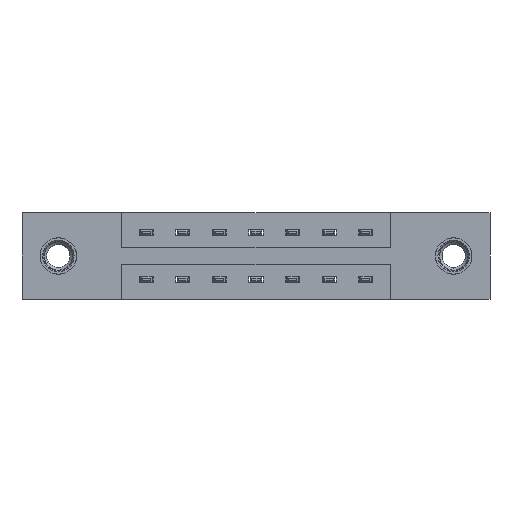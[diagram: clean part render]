
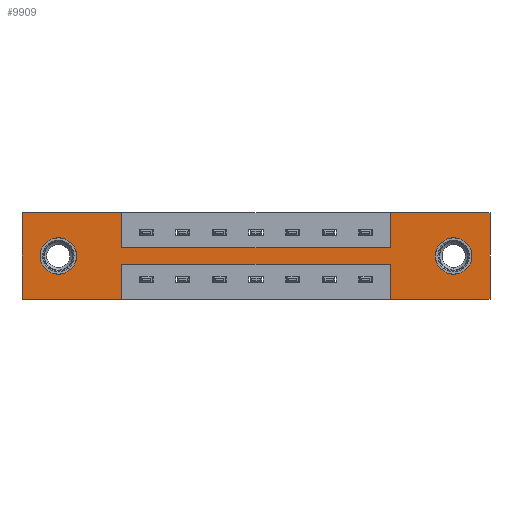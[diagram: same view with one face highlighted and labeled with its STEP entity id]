
A CAD part, front view. The second image highlights one B-rep face of the part: STEP entity #9909.
In plain terms, the highlighted planar face has unit normal (0, -1, 0).
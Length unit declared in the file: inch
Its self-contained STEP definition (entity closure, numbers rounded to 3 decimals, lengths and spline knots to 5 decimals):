
#42 = CARTESIAN_POINT ( 'NONE',  ( 0.425, 0., 0. ) ) ;
#105 = CARTESIAN_POINT ( 'NONE',  ( 1.843, 0., -0.263 ) ) ;
#265 = DIRECTION ( 'NONE',  ( 0., 0., 1. ) ) ;
#335 = DIRECTION ( 'NONE',  ( 0., 0., -1. ) ) ;
#348 = CARTESIAN_POINT ( 'NONE',  ( 0., 0., 0. ) ) ;
#365 = FACE_BOUND ( 'NONE', #8200, .T. ) ;
#426 = LINE ( 'NONE', #6497, #5454 ) ;
#581 = DIRECTION ( 'NONE',  ( 0., 0., 1. ) ) ;
#606 = EDGE_CURVE ( 'NONE', #2423, #4986, #8933, .T. ) ;
#896 = FACE_BOUND ( 'NONE', #5640, .T. ) ;
#1083 = VECTOR ( 'NONE', #9210, 39.37008 ) ;
#1389 = EDGE_CURVE ( 'NONE', #10096, #5776, #8411, .T. ) ;
#1401 = VERTEX_POINT ( 'NONE', #105 ) ;
#1419 = DIRECTION ( 'NONE',  ( 0., 0., -1. ) ) ;
#1502 = VECTOR ( 'NONE', #4473, 39.37008 ) ;
#1526 = CARTESIAN_POINT ( 'NONE',  ( 1.573, 0., -0.37 ) ) ;
#1586 = DIRECTION ( 'NONE',  ( 0., 1., 0. ) ) ;
#1689 = DIRECTION ( 'NONE',  ( 0., 0., -1. ) ) ;
#1734 = DIRECTION ( 'NONE',  ( 0., -1., 0. ) ) ;
#1774 = VERTEX_POINT ( 'NONE', #4088 ) ;
#1817 = PLANE ( 'NONE',  #8766 ) ;
#2056 = DIRECTION ( 'NONE',  ( -1., 0., 0. ) ) ;
#2137 = LINE ( 'NONE', #7655, #5462 ) ;
#2291 = EDGE_CURVE ( 'NONE', #4266, #7596, #2137, .T. ) ;
#2322 = CIRCLE ( 'NONE', #10658, 0.078 ) ;
#2397 = CARTESIAN_POINT ( 'NONE',  ( 0., 0., -0.37 ) ) ;
#2423 = VERTEX_POINT ( 'NONE', #4426 ) ;
#2525 = DIRECTION ( 'NONE',  ( 1., 0., 0. ) ) ;
#2531 = ORIENTED_EDGE ( 'NONE', *, *, #10396, .T. ) ;
#2560 = CARTESIAN_POINT ( 'NONE',  ( 0., 0., -0.37 ) ) ;
#2608 = EDGE_CURVE ( 'NONE', #10381, #10036, #426, .T. ) ;
#2638 = CARTESIAN_POINT ( 'NONE',  ( 1.843, 0., -0.185 ) ) ;
#2710 = ORIENTED_EDGE ( 'NONE', *, *, #8866, .T. ) ;
#2764 = CARTESIAN_POINT ( 'NONE',  ( 0., 0., -0.37 ) ) ;
#2765 = EDGE_CURVE ( 'NONE', #7596, #10561, #3045, .T. ) ;
#2774 = LINE ( 'NONE', #3293, #1083 ) ;
#2861 = FACE_OUTER_BOUND ( 'NONE', #7091, .T. ) ;
#2928 = DIRECTION ( 'NONE',  ( 0., 1., 0. ) ) ;
#3004 = CIRCLE ( 'NONE', #9980, 0.078 ) ;
#3045 = LINE ( 'NONE', #4150, #3320 ) ;
#3112 = ORIENTED_EDGE ( 'NONE', *, *, #2765, .F. ) ;
#3240 = ORIENTED_EDGE ( 'NONE', *, *, #10457, .F. ) ;
#3293 = CARTESIAN_POINT ( 'NONE',  ( 0.425, 0., -0.15 ) ) ;
#3320 = VECTOR ( 'NONE', #1689, 39.37008 ) ;
#3456 = EDGE_CURVE ( 'NONE', #5776, #10381, #4489, .T. ) ;
#3622 = DIRECTION ( 'NONE',  ( 0., 0., -1. ) ) ;
#3805 = EDGE_CURVE ( 'NONE', #10036, #6837, #9666, .T. ) ;
#3897 = CARTESIAN_POINT ( 'NONE',  ( 1.573, 0., -0.37 ) ) ;
#3996 = ORIENTED_EDGE ( 'NONE', *, *, #2608, .F. ) ;
#4067 = DIRECTION ( 'NONE',  ( 0., 0., 1. ) ) ;
#4088 = CARTESIAN_POINT ( 'NONE',  ( 1.573, 0., -0.22 ) ) ;
#4130 = EDGE_CURVE ( 'NONE', #7897, #1401, #2322, .T. ) ;
#4150 = CARTESIAN_POINT ( 'NONE',  ( 1.998, 0., 0. ) ) ;
#4266 = VERTEX_POINT ( 'NONE', #9884 ) ;
#4390 = DIRECTION ( 'NONE',  ( 0., 1., 0. ) ) ;
#4395 = DIRECTION ( 'NONE',  ( 0., 1., 0. ) ) ;
#4426 = CARTESIAN_POINT ( 'NONE',  ( 0.155, 0., -0.107 ) ) ;
#4473 = DIRECTION ( 'NONE',  ( -1., 0., 0. ) ) ;
#4476 = CARTESIAN_POINT ( 'NONE',  ( 0.155, 0., -0.263 ) ) ;
#4489 = LINE ( 'NONE', #2764, #8857 ) ;
#4522 = ORIENTED_EDGE ( 'NONE', *, *, #2291, .F. ) ;
#4548 = ORIENTED_EDGE ( 'NONE', *, *, #10184, .F. ) ;
#4585 = EDGE_CURVE ( 'NONE', #1774, #10096, #4837, .T. ) ;
#4681 = ORIENTED_EDGE ( 'NONE', *, *, #3456, .F. ) ;
#4739 = CARTESIAN_POINT ( 'NONE',  ( 1.998, 0., -0.37 ) ) ;
#4756 = CARTESIAN_POINT ( 'NONE',  ( 0.425, 0., -0.22 ) ) ;
#4837 = LINE ( 'NONE', #4756, #8295 ) ;
#4872 = DIRECTION ( 'NONE',  ( 0., 0., 1. ) ) ;
#4978 = EDGE_CURVE ( 'NONE', #8568, #4266, #10129, .T. ) ;
#4986 = VERTEX_POINT ( 'NONE', #4476 ) ;
#5017 = VECTOR ( 'NONE', #4067, 39.37008 ) ;
#5087 = CARTESIAN_POINT ( 'NONE',  ( 0.155, 0., -0.185 ) ) ;
#5210 = VECTOR ( 'NONE', #6815, 39.37008 ) ;
#5211 = CIRCLE ( 'NONE', #9772, 0.078 ) ;
#5296 = CARTESIAN_POINT ( 'NONE',  ( 1.843, 0., -0.185 ) ) ;
#5454 = VECTOR ( 'NONE', #4872, 39.37008 ) ;
#5462 = VECTOR ( 'NONE', #2525, 39.37008 ) ;
#5640 = EDGE_LOOP ( 'NONE', ( #6501, #2531 ) ) ;
#5776 = VERTEX_POINT ( 'NONE', #7978 ) ;
#6069 = CARTESIAN_POINT ( 'NONE',  ( 1.573, 0., 0. ) ) ;
#6083 = VECTOR ( 'NONE', #9700, 39.37008 ) ;
#6188 = DIRECTION ( 'NONE',  ( -1., 0., 0. ) ) ;
#6310 = CARTESIAN_POINT ( 'NONE',  ( 0.155, 0., -0.185 ) ) ;
#6323 = ORIENTED_EDGE ( 'NONE', *, *, #1389, .F. ) ;
#6360 = AXIS2_PLACEMENT_3D ( 'NONE', #6310, #2928, #581 ) ;
#6497 = CARTESIAN_POINT ( 'NONE',  ( 0., 0., 0. ) ) ;
#6501 = ORIENTED_EDGE ( 'NONE', *, *, #4130, .T. ) ;
#6815 = DIRECTION ( 'NONE',  ( 0., 0., -1. ) ) ;
#6837 = VERTEX_POINT ( 'NONE', #42 ) ;
#7091 = EDGE_LOOP ( 'NONE', ( #6323, #9932, #8326, #3240, #3112, #4522, #8718, #7774, #4548, #9928, #3996, #4681 ) ) ;
#7114 = ORIENTED_EDGE ( 'NONE', *, *, #606, .T. ) ;
#7268 = LINE ( 'NONE', #1526, #5017 ) ;
#7463 = CARTESIAN_POINT ( 'NONE',  ( 0., 0., 0. ) ) ;
#7466 = EDGE_CURVE ( 'NONE', #9577, #8568, #2774, .T. ) ;
#7534 = VERTEX_POINT ( 'NONE', #3897 ) ;
#7596 = VERTEX_POINT ( 'NONE', #10694 ) ;
#7630 = DIRECTION ( 'NONE',  ( 0., 0., 1. ) ) ;
#7655 = CARTESIAN_POINT ( 'NONE',  ( 0., 0., 0. ) ) ;
#7656 = DIRECTION ( 'NONE',  ( 0., 0., -1. ) ) ;
#7774 = ORIENTED_EDGE ( 'NONE', *, *, #7466, .F. ) ;
#7897 = VERTEX_POINT ( 'NONE', #10203 ) ;
#7978 = CARTESIAN_POINT ( 'NONE',  ( 0.425, 0., -0.37 ) ) ;
#8200 = EDGE_LOOP ( 'NONE', ( #7114, #2710 ) ) ;
#8248 = CARTESIAN_POINT ( 'NONE',  ( 0.425, 0., 0. ) ) ;
#8295 = VECTOR ( 'NONE', #2056, 39.37008 ) ;
#8326 = ORIENTED_EDGE ( 'NONE', *, *, #8831, .F. ) ;
#8411 = LINE ( 'NONE', #10877, #5210 ) ;
#8568 = VERTEX_POINT ( 'NONE', #8579 ) ;
#8579 = CARTESIAN_POINT ( 'NONE',  ( 1.573, 0., -0.15 ) ) ;
#8635 = VECTOR ( 'NONE', #1419, 39.37008 ) ;
#8718 = ORIENTED_EDGE ( 'NONE', *, *, #4978, .F. ) ;
#8765 = LINE ( 'NONE', #8248, #8635 ) ;
#8766 = AXIS2_PLACEMENT_3D ( 'NONE', #2560, #1734, #7656 ) ;
#8831 = EDGE_CURVE ( 'NONE', #7534, #1774, #7268, .T. ) ;
#8857 = VECTOR ( 'NONE', #6188, 39.37008 ) ;
#8866 = EDGE_CURVE ( 'NONE', #4986, #2423, #3004, .T. ) ;
#8925 = VECTOR ( 'NONE', #265, 39.37008 ) ;
#8933 = CIRCLE ( 'NONE', #6360, 0.078 ) ;
#9210 = DIRECTION ( 'NONE',  ( 1., 0., 0. ) ) ;
#9577 = VERTEX_POINT ( 'NONE', #10891 ) ;
#9666 = LINE ( 'NONE', #348, #6083 ) ;
#9700 = DIRECTION ( 'NONE',  ( 1., 0., 0. ) ) ;
#9708 = LINE ( 'NONE', #10363, #1502 ) ;
#9772 = AXIS2_PLACEMENT_3D ( 'NONE', #2638, #4395, #3622 ) ;
#9884 = CARTESIAN_POINT ( 'NONE',  ( 1.573, 0., 0. ) ) ;
#9909 = ADVANCED_FACE ( 'NONE', ( #896, #365, #2861 ), #1817, .T. ) ;
#9928 = ORIENTED_EDGE ( 'NONE', *, *, #3805, .F. ) ;
#9932 = ORIENTED_EDGE ( 'NONE', *, *, #4585, .F. ) ;
#9980 = AXIS2_PLACEMENT_3D ( 'NONE', #5087, #1586, #7630 ) ;
#10036 = VERTEX_POINT ( 'NONE', #7463 ) ;
#10096 = VERTEX_POINT ( 'NONE', #10601 ) ;
#10129 = LINE ( 'NONE', #6069, #8925 ) ;
#10184 = EDGE_CURVE ( 'NONE', #6837, #9577, #8765, .T. ) ;
#10203 = CARTESIAN_POINT ( 'NONE',  ( 1.843, 0., -0.107 ) ) ;
#10363 = CARTESIAN_POINT ( 'NONE',  ( 0., 0., -0.37 ) ) ;
#10381 = VERTEX_POINT ( 'NONE', #2397 ) ;
#10396 = EDGE_CURVE ( 'NONE', #1401, #7897, #5211, .T. ) ;
#10457 = EDGE_CURVE ( 'NONE', #10561, #7534, #9708, .T. ) ;
#10561 = VERTEX_POINT ( 'NONE', #4739 ) ;
#10601 = CARTESIAN_POINT ( 'NONE',  ( 0.425, 0., -0.22 ) ) ;
#10658 = AXIS2_PLACEMENT_3D ( 'NONE', #5296, #4390, #335 ) ;
#10694 = CARTESIAN_POINT ( 'NONE',  ( 1.998, 0., 0. ) ) ;
#10877 = CARTESIAN_POINT ( 'NONE',  ( 0.425, 0., -0.37 ) ) ;
#10891 = CARTESIAN_POINT ( 'NONE',  ( 0.425, 0., -0.15 ) ) ;
